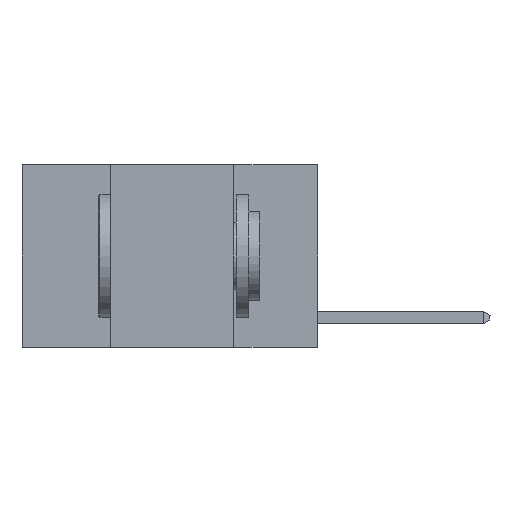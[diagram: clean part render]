
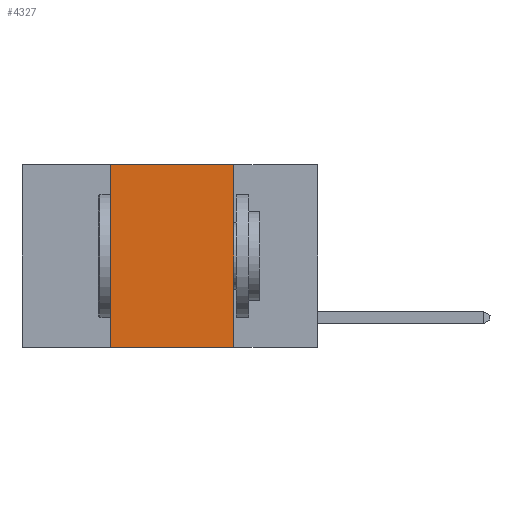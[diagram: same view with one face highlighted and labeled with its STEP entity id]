
A CAD part, left-side view. The second image highlights one B-rep face of the part: STEP entity #4327.
In plain terms, the highlighted planar face has unit normal (-1, 0, 0).
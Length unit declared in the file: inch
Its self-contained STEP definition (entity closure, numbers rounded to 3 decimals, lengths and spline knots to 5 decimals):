
#116 = ORIENTED_EDGE ( 'NONE', *, *, #11075, .T. ) ;
#330 = PLANE ( 'NONE',  #6860 ) ;
#521 = ORIENTED_EDGE ( 'NONE', *, *, #10125, .F. ) ;
#1220 = ORIENTED_EDGE ( 'NONE', *, *, #2380, .F. ) ;
#1312 = DIRECTION ( 'NONE',  ( 0., 0., -1. ) ) ;
#1508 = CARTESIAN_POINT ( 'NONE',  ( 0., 0.42, 0. ) ) ;
#1978 = DIRECTION ( 'NONE',  ( 0., 0., -1. ) ) ;
#2142 = VERTEX_POINT ( 'NONE', #9009 ) ;
#2380 = EDGE_CURVE ( 'NONE', #9139, #11003, #9705, .T. ) ;
#3221 = CARTESIAN_POINT ( 'NONE',  ( 0., 0.6, 0. ) ) ;
#4327 = ADVANCED_FACE ( 'NONE', ( #6467 ), #330, .F. ) ;
#4694 = VERTEX_POINT ( 'NONE', #10338 ) ;
#4851 = ORIENTED_EDGE ( 'NONE', *, *, #9456, .F. ) ;
#5026 = DIRECTION ( 'NONE',  ( 0., -1., 0. ) ) ;
#5265 = CARTESIAN_POINT ( 'NONE',  ( 0., 0.6, 0. ) ) ;
#6220 = DIRECTION ( 'NONE',  ( 0., -1., 0. ) ) ;
#6467 = FACE_OUTER_BOUND ( 'NONE', #9624, .T. ) ;
#6860 = AXIS2_PLACEMENT_3D ( 'NONE', #3221, #7042, #1312 ) ;
#7042 = DIRECTION ( 'NONE',  ( 1., 0., 0. ) ) ;
#7240 = VECTOR ( 'NONE', #1978, 39.37008 ) ;
#7244 = DIRECTION ( 'NONE',  ( 0., 0., 1. ) ) ;
#7613 = CARTESIAN_POINT ( 'NONE',  ( 0., 0.17, 0. ) ) ;
#7668 = LINE ( 'NONE', #5265, #9268 ) ;
#8489 = VECTOR ( 'NONE', #5026, 39.37008 ) ;
#8894 = CARTESIAN_POINT ( 'NONE',  ( 0., 0.17, 0. ) ) ;
#9009 = CARTESIAN_POINT ( 'NONE',  ( 0., 0.42, 0. ) ) ;
#9139 = VERTEX_POINT ( 'NONE', #7613 ) ;
#9268 = VECTOR ( 'NONE', #6220, 39.37008 ) ;
#9456 = EDGE_CURVE ( 'NONE', #2142, #9139, #7668, .T. ) ;
#9624 = EDGE_LOOP ( 'NONE', ( #1220, #4851, #521, #116 ) ) ;
#9705 = LINE ( 'NONE', #8894, #7240 ) ;
#10125 = EDGE_CURVE ( 'NONE', #4694, #2142, #11887, .T. ) ;
#10338 = CARTESIAN_POINT ( 'NONE',  ( 0., 0.42, -0.37 ) ) ;
#10647 = CARTESIAN_POINT ( 'NONE',  ( 0., 0.6, -0.37 ) ) ;
#10696 = LINE ( 'NONE', #10647, #8489 ) ;
#11003 = VERTEX_POINT ( 'NONE', #11462 ) ;
#11075 = EDGE_CURVE ( 'NONE', #4694, #11003, #10696, .T. ) ;
#11462 = CARTESIAN_POINT ( 'NONE',  ( 0., 0.17, -0.37 ) ) ;
#11887 = LINE ( 'NONE', #1508, #12171 ) ;
#12171 = VECTOR ( 'NONE', #7244, 39.37008 ) ;
